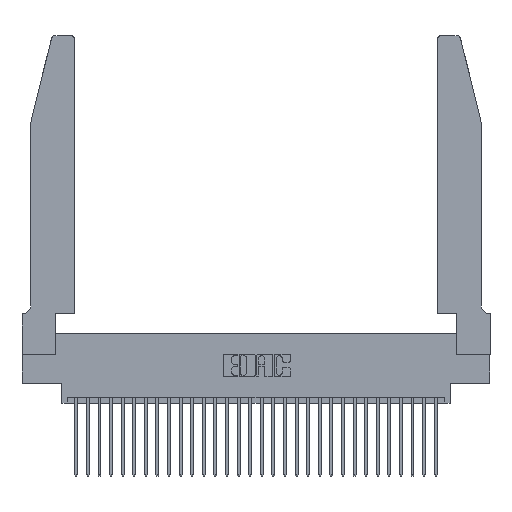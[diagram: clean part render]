
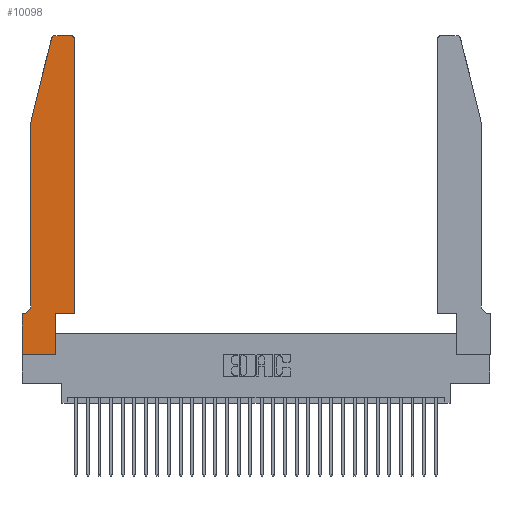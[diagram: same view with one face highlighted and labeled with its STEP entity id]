
A CAD part, top view. The second image highlights one B-rep face of the part: STEP entity #10098.
In plain terms, the highlighted planar face has unit normal (0, 0, 1).
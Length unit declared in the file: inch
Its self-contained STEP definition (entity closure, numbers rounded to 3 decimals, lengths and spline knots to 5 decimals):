
#58 = VECTOR ( 'NONE', #16641, 39.37008 ) ;
#341 = ORIENTED_EDGE ( 'NONE', *, *, #31201, .T. ) ;
#705 = VECTOR ( 'NONE', #15191, 39.37008 ) ;
#825 = ORIENTED_EDGE ( 'NONE', *, *, #22126, .T. ) ;
#1197 = CARTESIAN_POINT ( 'NONE',  ( 0.25487, 2.72718, 0.37 ) ) ;
#1626 = VECTOR ( 'NONE', #14551, 39.37008 ) ;
#1769 = ORIENTED_EDGE ( 'NONE', *, *, #29576, .T. ) ;
#1984 = VECTOR ( 'NONE', #20159, 39.37008 ) ;
#2356 = ORIENTED_EDGE ( 'NONE', *, *, #14900, .T. ) ;
#2546 = AXIS2_PLACEMENT_3D ( 'NONE', #10485, #27316, #12904 ) ;
#2761 = ORIENTED_EDGE ( 'NONE', *, *, #27772, .T. ) ;
#2859 = ORIENTED_EDGE ( 'NONE', *, *, #7233, .T. ) ;
#3000 = DIRECTION ( 'NONE',  ( 0., 0., 1. ) ) ;
#3023 = LINE ( 'NONE', #17532, #705 ) ;
#3252 = CARTESIAN_POINT ( 'NONE',  ( 0.284, 2.72, 0.37 ) ) ;
#3305 = ORIENTED_EDGE ( 'NONE', *, *, #5541, .T. ) ;
#3817 = EDGE_LOOP ( 'NONE', ( #341, #825, #1769, #2356, #2761, #2859, #3305, #3828, #4610, #4885, #5042, #6025 ) ) ;
#3828 = ORIENTED_EDGE ( 'NONE', *, *, #28513, .T. ) ;
#4219 = CARTESIAN_POINT ( 'NONE',  ( 0., 0., 0.37 ) ) ;
#4461 = CIRCLE ( 'NONE', #2546, 0.03 ) ;
#4610 = ORIENTED_EDGE ( 'NONE', *, *, #19122, .T. ) ;
#4885 = ORIENTED_EDGE ( 'NONE', *, *, #10210, .T. ) ;
#5030 = CIRCLE ( 'NONE', #27675, 0.03 ) ;
#5042 = ORIENTED_EDGE ( 'NONE', *, *, #5311, .T. ) ;
#5311 = EDGE_CURVE ( 'NONE', #25183, #25187, #8242, .T. ) ;
#5541 = EDGE_CURVE ( 'NONE', #28019, #19109, #15023, .T. ) ;
#5603 = CARTESIAN_POINT ( 'NONE',  ( 0., 0., 0.37 ) ) ;
#5760 = DIRECTION ( 'NONE',  ( 1., 0., 0. ) ) ;
#6025 = ORIENTED_EDGE ( 'NONE', *, *, #31047, .T. ) ;
#6213 = CARTESIAN_POINT ( 'NONE',  ( 0.2605, 2.75, 0.37 ) ) ;
#6388 = VECTOR ( 'NONE', #20755, 39.37008 ) ;
#6699 = LINE ( 'NONE', #14205, #58 ) ;
#6879 = CARTESIAN_POINT ( 'NONE',  ( 0., 0., 0.37 ) ) ;
#7233 = EDGE_CURVE ( 'NONE', #12217, #28019, #18734, .T. ) ;
#7259 = CARTESIAN_POINT ( 'NONE',  ( 0., 0.35, 0.37 ) ) ;
#7646 = LINE ( 'NONE', #27843, #19784 ) ;
#7747 = VERTEX_POINT ( 'NONE', #9054 ) ;
#8242 = LINE ( 'NONE', #21722, #1626 ) ;
#9054 = CARTESIAN_POINT ( 'NONE',  ( 0.284, 2.75, 0.37 ) ) ;
#9247 = VECTOR ( 'NONE', #25617, 39.37008 ) ;
#9310 = VERTEX_POINT ( 'NONE', #14608 ) ;
#9991 = LINE ( 'NONE', #25072, #9247 ) ;
#10098 = ADVANCED_FACE ( 'NONE', ( #13011 ), #29541, .T. ) ;
#10210 = EDGE_CURVE ( 'NONE', #11273, #25183, #9991, .T. ) ;
#10436 = CARTESIAN_POINT ( 'NONE',  ( 0.0055, 0.35, 0.37 ) ) ;
#10485 = CARTESIAN_POINT ( 'NONE',  ( 0.4205, 2.72, 0.37 ) ) ;
#11025 = DIRECTION ( 'NONE',  ( -0.239, -0.971, 0. ) ) ;
#11273 = VERTEX_POINT ( 'NONE', #20659 ) ;
#12217 = VERTEX_POINT ( 'NONE', #10436 ) ;
#12904 = DIRECTION ( 'NONE',  ( 1., 0., 0. ) ) ;
#13011 = FACE_OUTER_BOUND ( 'NONE', #3817, .T. ) ;
#13625 = CARTESIAN_POINT ( 'NONE',  ( 0.0055, 0.42, 0.37 ) ) ;
#14205 = CARTESIAN_POINT ( 'NONE',  ( 0.2865, 0.35, 0.37 ) ) ;
#14447 = CARTESIAN_POINT ( 'NONE',  ( 0.0755, 0.35, 0.37 ) ) ;
#14535 = VERTEX_POINT ( 'NONE', #1197 ) ;
#14539 = CIRCLE ( 'NONE', #27088, 0.07 ) ;
#14551 = DIRECTION ( 'NONE',  ( 0., 1., 0. ) ) ;
#14608 = CARTESIAN_POINT ( 'NONE',  ( 0.4205, 2.75, 0.37 ) ) ;
#14623 = CARTESIAN_POINT ( 'NONE',  ( 0.4505, 0.35, 0.37 ) ) ;
#14900 = EDGE_CURVE ( 'NONE', #26006, #19039, #3023, .T. ) ;
#14988 = CARTESIAN_POINT ( 'NONE',  ( 0., 0.35, 0.37 ) ) ;
#15023 = LINE ( 'NONE', #5603, #1984 ) ;
#15191 = DIRECTION ( 'NONE',  ( 0., -1., 0. ) ) ;
#16056 = DIRECTION ( 'NONE',  ( -1., 0., 0. ) ) ;
#16641 = DIRECTION ( 'NONE',  ( 0., 1., 0. ) ) ;
#17532 = CARTESIAN_POINT ( 'NONE',  ( 0.0755, 2., 0.37 ) ) ;
#18550 = LINE ( 'NONE', #6213, #6388 ) ;
#18734 = LINE ( 'NONE', #14447, #25842 ) ;
#19039 = VERTEX_POINT ( 'NONE', #28382 ) ;
#19109 = VERTEX_POINT ( 'NONE', #6879 ) ;
#19122 = EDGE_CURVE ( 'NONE', #28674, #11273, #6699, .T. ) ;
#19784 = VECTOR ( 'NONE', #11025, 39.37008 ) ;
#20071 = DIRECTION ( 'NONE',  ( 1., 0., 0. ) ) ;
#20159 = DIRECTION ( 'NONE',  ( 0., -1., 0. ) ) ;
#20315 = DIRECTION ( 'NONE',  ( 0., 0., 1. ) ) ;
#20659 = CARTESIAN_POINT ( 'NONE',  ( 0.2865, 0.35, 0.37 ) ) ;
#20755 = DIRECTION ( 'NONE',  ( -1., 0., 0. ) ) ;
#21224 = DIRECTION ( 'NONE',  ( 1., 0., 0. ) ) ;
#21722 = CARTESIAN_POINT ( 'NONE',  ( 0.4505, 0.35, 0.37 ) ) ;
#22126 = EDGE_CURVE ( 'NONE', #7747, #14535, #5030, .T. ) ;
#24470 = AXIS2_PLACEMENT_3D ( 'NONE', #14988, #3000, #20071 ) ;
#24648 = VECTOR ( 'NONE', #21224, 39.37008 ) ;
#25072 = CARTESIAN_POINT ( 'NONE',  ( 0.4505, 0.35, 0.37 ) ) ;
#25183 = VERTEX_POINT ( 'NONE', #14623 ) ;
#25187 = VERTEX_POINT ( 'NONE', #26590 ) ;
#25617 = DIRECTION ( 'NONE',  ( 1., 0., 0. ) ) ;
#25842 = VECTOR ( 'NONE', #31189, 39.37008 ) ;
#26006 = VERTEX_POINT ( 'NONE', #30289 ) ;
#26590 = CARTESIAN_POINT ( 'NONE',  ( 0.4505, 2.72, 0.37 ) ) ;
#27088 = AXIS2_PLACEMENT_3D ( 'NONE', #13625, #30402, #16056 ) ;
#27316 = DIRECTION ( 'NONE',  ( 0., 0., 1. ) ) ;
#27675 = AXIS2_PLACEMENT_3D ( 'NONE', #3252, #20315, #5760 ) ;
#27772 = EDGE_CURVE ( 'NONE', #19039, #12217, #14539, .T. ) ;
#27843 = CARTESIAN_POINT ( 'NONE',  ( 0.0755, 2., 0.37 ) ) ;
#28019 = VERTEX_POINT ( 'NONE', #7259 ) ;
#28382 = CARTESIAN_POINT ( 'NONE',  ( 0.0755, 0.42, 0.37 ) ) ;
#28513 = EDGE_CURVE ( 'NONE', #19109, #28674, #30244, .T. ) ;
#28674 = VERTEX_POINT ( 'NONE', #28887 ) ;
#28887 = CARTESIAN_POINT ( 'NONE',  ( 0.2865, 0., 0.37 ) ) ;
#29541 = PLANE ( 'NONE',  #24470 ) ;
#29576 = EDGE_CURVE ( 'NONE', #14535, #26006, #7646, .T. ) ;
#30244 = LINE ( 'NONE', #4219, #24648 ) ;
#30289 = CARTESIAN_POINT ( 'NONE',  ( 0.0755, 2., 0.37 ) ) ;
#30402 = DIRECTION ( 'NONE',  ( 0., 0., -1. ) ) ;
#31047 = EDGE_CURVE ( 'NONE', #25187, #9310, #4461, .T. ) ;
#31189 = DIRECTION ( 'NONE',  ( -1., 0., 0. ) ) ;
#31201 = EDGE_CURVE ( 'NONE', #9310, #7747, #18550, .T. ) ;
